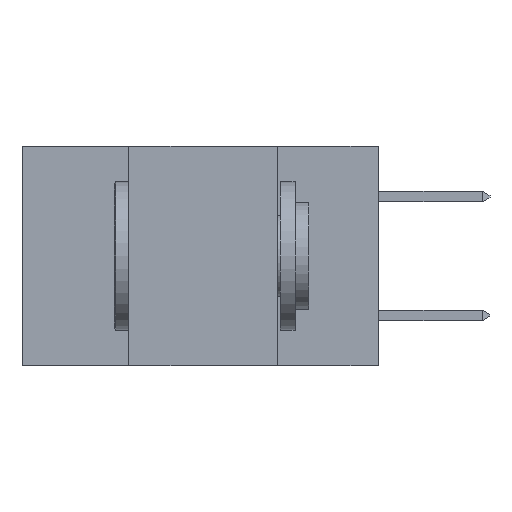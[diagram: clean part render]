
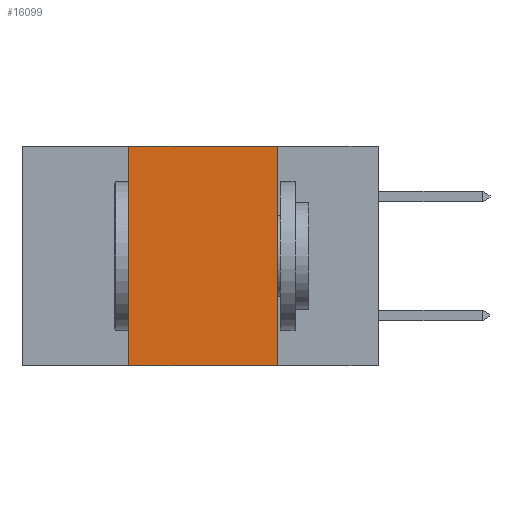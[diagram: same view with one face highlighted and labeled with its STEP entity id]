
A CAD part, left-side view. The second image highlights one B-rep face of the part: STEP entity #16099.
In plain terms, the highlighted planar face has unit normal (-1, 0, 0).
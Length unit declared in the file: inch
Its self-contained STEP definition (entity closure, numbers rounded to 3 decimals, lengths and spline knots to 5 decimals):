
#251 = CARTESIAN_POINT ( 'NONE',  ( 0., 0.6, 0. ) ) ;
#785 = DIRECTION ( 'NONE',  ( 0., -1., 0. ) ) ;
#1352 = EDGE_CURVE ( 'NONE', #17684, #13941, #15987, .T. ) ;
#1712 = DIRECTION ( 'NONE',  ( 0., 0., -1. ) ) ;
#2310 = EDGE_CURVE ( 'NONE', #7423, #10175, #17435, .T. ) ;
#3481 = ORIENTED_EDGE ( 'NONE', *, *, #1352, .F. ) ;
#3580 = CARTESIAN_POINT ( 'NONE',  ( 0., 0.17, 0. ) ) ;
#4293 = DIRECTION ( 'NONE',  ( 0., 0., 1. ) ) ;
#5113 = CARTESIAN_POINT ( 'NONE',  ( 0., 0.6, 0. ) ) ;
#5134 = CARTESIAN_POINT ( 'NONE',  ( 0., 0.6, -0.37 ) ) ;
#5592 = ORIENTED_EDGE ( 'NONE', *, *, #2310, .F. ) ;
#7423 = VERTEX_POINT ( 'NONE', #3580 ) ;
#7450 = CARTESIAN_POINT ( 'NONE',  ( 0., 0.42, 0. ) ) ;
#8099 = CARTESIAN_POINT ( 'NONE',  ( 0., 0.17, 0. ) ) ;
#8143 = DIRECTION ( 'NONE',  ( 0., 0., -1. ) ) ;
#9121 = PLANE ( 'NONE',  #9221 ) ;
#9221 = AXIS2_PLACEMENT_3D ( 'NONE', #251, #10656, #1712 ) ;
#9432 = EDGE_CURVE ( 'NONE', #13941, #7423, #17576, .T. ) ;
#10149 = LINE ( 'NONE', #5134, #13902 ) ;
#10175 = VERTEX_POINT ( 'NONE', #17942 ) ;
#10656 = DIRECTION ( 'NONE',  ( 1., 0., 0. ) ) ;
#10723 = FACE_OUTER_BOUND ( 'NONE', #10940, .T. ) ;
#10940 = EDGE_LOOP ( 'NONE', ( #5592, #17031, #3481, #15985 ) ) ;
#13902 = VECTOR ( 'NONE', #785, 39.37008 ) ;
#13941 = VERTEX_POINT ( 'NONE', #15144 ) ;
#14343 = VECTOR ( 'NONE', #15268, 39.37008 ) ;
#15122 = VECTOR ( 'NONE', #4293, 39.37008 ) ;
#15144 = CARTESIAN_POINT ( 'NONE',  ( 0., 0.42, 0. ) ) ;
#15268 = DIRECTION ( 'NONE',  ( 0., -1., 0. ) ) ;
#15653 = CARTESIAN_POINT ( 'NONE',  ( 0., 0.42, -0.37 ) ) ;
#15985 = ORIENTED_EDGE ( 'NONE', *, *, #18123, .T. ) ;
#15987 = LINE ( 'NONE', #7450, #15122 ) ;
#16099 = ADVANCED_FACE ( 'NONE', ( #10723 ), #9121, .F. ) ;
#16995 = VECTOR ( 'NONE', #8143, 39.37008 ) ;
#17031 = ORIENTED_EDGE ( 'NONE', *, *, #9432, .F. ) ;
#17435 = LINE ( 'NONE', #8099, #16995 ) ;
#17576 = LINE ( 'NONE', #5113, #14343 ) ;
#17684 = VERTEX_POINT ( 'NONE', #15653 ) ;
#17942 = CARTESIAN_POINT ( 'NONE',  ( 0., 0.17, -0.37 ) ) ;
#18123 = EDGE_CURVE ( 'NONE', #17684, #10175, #10149, .T. ) ;
